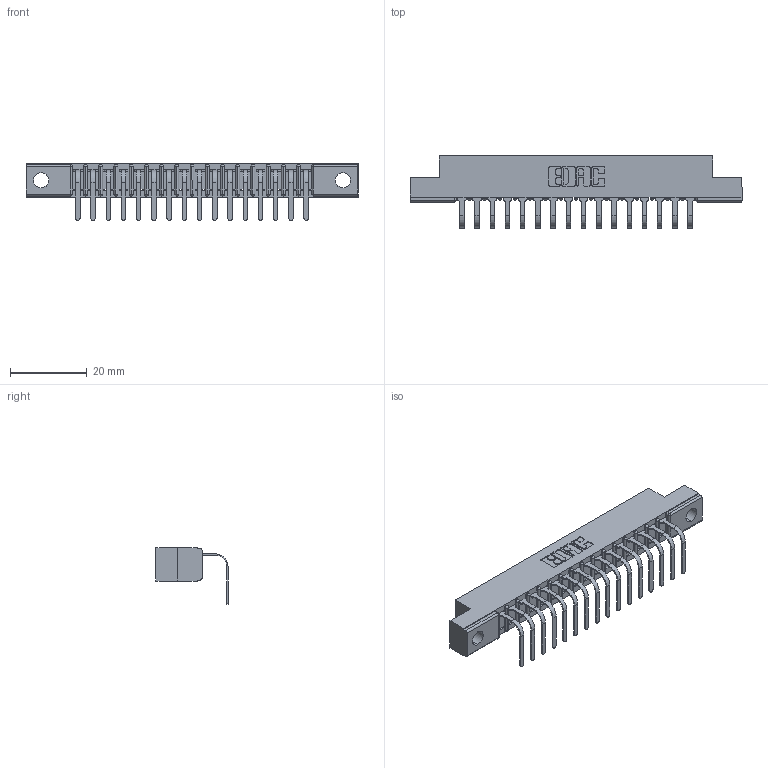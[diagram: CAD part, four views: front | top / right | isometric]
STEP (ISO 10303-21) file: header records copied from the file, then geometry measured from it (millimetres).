
FILE_DESCRIPTION (( 'STEP AP203' ), '1' );
FILE_NAME ('357-016-458-102.STEP', '2022-07-18T23:10:41', ( '' ), ( '' ), 'SwSTEP 2.0', 'SolidWorks 2020', '' );
FILE_SCHEMA (( 'CONFIG_CONTROL_DESIGN' ));
Length unit declared in the file: inch
Products named in the file (3): 357-016-458-102; 307 Part_.128 Dia Mounting Holes; 307-290-001_558 - 2 (Single)
Assembly tree (17 placements, depth 2):
  357-016-458-102
    307 Part_.128 Dia Mounting Holes
    307-290-001_558 - 2 (Single)  x16
Bounding box: 86.41 x 18.78 x 14.81 mm (x, y, z)
Volume: 5448.6 mm3; surface area: 8452.6 mm2
Topology: 17 solids, 17 shells, 1095 faces, 3107 edges, 2002 vertices
Faces by surface type: plane 694, cylinder 367, sphere 34
Entity records: 17028 total; most frequent: CARTESIAN_POINT 2860, ORIENTED_EDGE 2846, DIRECTION 2797, EDGE_CURVE 1423, VECTOR 1079, LINE 1079, VERTEX_POINT 922, AXIS2_PLACEMENT_3D 859
